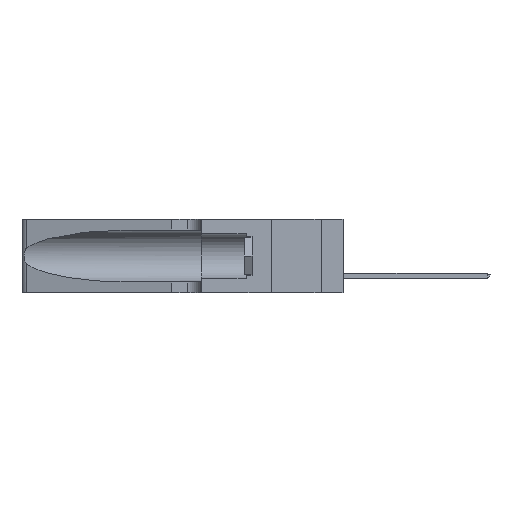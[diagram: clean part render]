
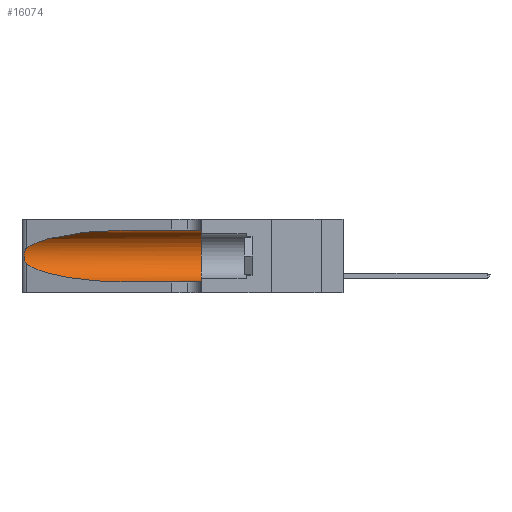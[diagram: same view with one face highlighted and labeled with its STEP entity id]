
A CAD part, left-side view. The second image highlights one B-rep face of the part: STEP entity #16074.
In plain terms, the highlighted cylindrical face has radius 3.308 mm (diameter 6.617 mm), a partial arc.
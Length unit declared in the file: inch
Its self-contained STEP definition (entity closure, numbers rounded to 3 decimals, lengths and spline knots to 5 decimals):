
#273 = CARTESIAN_POINT ( 'NONE',  ( 0.1305, 0.72297, 0.31525 ) ) ;
#564 = DIRECTION ( 'NONE',  ( 0., -1., 0. ) ) ;
#1654 = ORIENTED_EDGE ( 'NONE', *, *, #5495, .T. ) ;
#1999 = ORIENTED_EDGE ( 'NONE', *, *, #29885, .T. ) ;
#2245 = CARTESIAN_POINT ( 'NONE',  ( 0.25487, 1.22718, 0.14631 ) ) ;
#2535 = DIRECTION ( 'NONE',  ( 0., 0., 1. ) ) ;
#2566 = VERTEX_POINT ( 'NONE', #273 ) ;
#2699 = FACE_OUTER_BOUND ( 'NONE', #11051, .T. ) ;
#2924 = ORIENTED_EDGE ( 'NONE', *, *, #5559, .T. ) ;
#2955 = B_SPLINE_CURVE_WITH_KNOTS ( 'NONE', 3,
 ( #9701, #29972, #27235, #32277, #24946, #12218, #29869, #29764, #32486, #17508, #22674, #14862, #32379, #2245 ),
 .UNSPECIFIED., .F., .F.,
 ( 4, 2, 2, 2, 2, 2, 4 ),
 ( 0., 0.00027, 0.00053, 0.00107, 0.0016, 0.00187, 0.00214 ),
 .UNSPECIFIED. ) ;
#3397 = VERTEX_POINT ( 'NONE', #14533 ) ;
#4637 = EDGE_CURVE ( 'NONE', #3397, #16923, #11590, .T. ) ;
#5464 = CARTESIAN_POINT ( 'NONE',  ( 0.1305, 1.61858, 0.05475 ) ) ;
#5495 = EDGE_CURVE ( 'NONE', #12617, #23636, #2955, .T. ) ;
#5559 = EDGE_CURVE ( 'NONE', #23636, #8234, #9598, .T. ) ;
#6628 = EDGE_CURVE ( 'NONE', #2566, #12617, #17271, .T. ) ;
#6962 = CARTESIAN_POINT ( 'NONE',  ( 0.25487, 1.22718, 0.14631 ) ) ;
#7368 = ORIENTED_EDGE ( 'NONE', *, *, #6628, .T. ) ;
#8213 = VECTOR ( 'NONE', #564, 39.37008 ) ;
#8224 = LINE ( 'NONE', #31324, #26681 ) ;
#8234 = VERTEX_POINT ( 'NONE', #17272 ) ;
#8596 = ORIENTED_EDGE ( 'NONE', *, *, #4637, .F. ) ;
#8785 = CARTESIAN_POINT ( 'NONE',  ( 0.1305, 1.61858, 0.185 ) ) ;
#9102 = CARTESIAN_POINT ( 'NONE',  ( 0.25487, 1.22718, 0.22369 ) ) ;
#9598 =( BOUNDED_CURVE ( )  B_SPLINE_CURVE ( 3, ( #6962, #16991, #24649, #24552 ),
 .UNSPECIFIED., .F., .T. ) 
 B_SPLINE_CURVE_WITH_KNOTS ( ( 4, 4 ),
 ( 3.44316, 4.71239 ),
 .UNSPECIFIED. ) 
 CURVE ( )  GEOMETRIC_REPRESENTATION_ITEM ( )  RATIONAL_B_SPLINE_CURVE ( ( 1., 0.87, 0.87, 1. ) ) 
 REPRESENTATION_ITEM ( '' )  );
#9701 = CARTESIAN_POINT ( 'NONE',  ( 0.25487, 1.22718, 0.22369 ) ) ;
#11051 = EDGE_LOOP ( 'NONE', ( #7368, #1654, #2924, #1999, #8596, #26667 ) ) ;
#11590 = CIRCLE ( 'NONE', #21489, 0.13025 ) ;
#12218 = CARTESIAN_POINT ( 'NONE',  ( 0.26018, 1.23835, 0.19895 ) ) ;
#12264 = CARTESIAN_POINT ( 'NONE',  ( 0.2373, 1.15595, 0.28018 ) ) ;
#12617 = VERTEX_POINT ( 'NONE', #29669 ) ;
#14064 = DIRECTION ( 'NONE',  ( 0., 0., -1. ) ) ;
#14533 = CARTESIAN_POINT ( 'NONE',  ( 0.1305, 0.35, 0.31525 ) ) ;
#14862 = CARTESIAN_POINT ( 'NONE',  ( 0.25639, 1.23186, 0.15144 ) ) ;
#14901 = LINE ( 'NONE', #5464, #8213 ) ;
#15504 = EDGE_CURVE ( 'NONE', #2566, #3397, #8224, .T. ) ;
#16074 = ADVANCED_FACE ( 'NONE', ( #2699 ), #27773, .F. ) ;
#16923 = VERTEX_POINT ( 'NONE', #26718 ) ;
#16991 = CARTESIAN_POINT ( 'NONE',  ( 0.2373, 1.15595, 0.08982 ) ) ;
#17271 =( BOUNDED_CURVE ( )  B_SPLINE_CURVE ( 3, ( #24604, #31240, #12264, #9102 ),
 .UNSPECIFIED., .F., .T. ) 
 B_SPLINE_CURVE_WITH_KNOTS ( ( 4, 4 ),
 ( 1.5708, 2.84003 ),
 .UNSPECIFIED. ) 
 CURVE ( )  GEOMETRIC_REPRESENTATION_ITEM ( )  RATIONAL_B_SPLINE_CURVE ( ( 1., 0.87, 0.87, 1. ) ) 
 REPRESENTATION_ITEM ( '' )  );
#17272 = CARTESIAN_POINT ( 'NONE',  ( 0.1305, 0.72297, 0.05475 ) ) ;
#17508 = CARTESIAN_POINT ( 'NONE',  ( 0.25856, 1.23593, 0.16098 ) ) ;
#17803 = DIRECTION ( 'NONE',  ( 0., 1., 0. ) ) ;
#18982 = DIRECTION ( 'NONE',  ( 0., -1., 0. ) ) ;
#21489 = AXIS2_PLACEMENT_3D ( 'NONE', #30247, #17803, #2535 ) ;
#22674 = CARTESIAN_POINT ( 'NONE',  ( 0.25789, 1.23486, 0.15765 ) ) ;
#23636 = VERTEX_POINT ( 'NONE', #26754 ) ;
#24552 = CARTESIAN_POINT ( 'NONE',  ( 0.1305, 0.72297, 0.05475 ) ) ;
#24604 = CARTESIAN_POINT ( 'NONE',  ( 0.1305, 0.72297, 0.31525 ) ) ;
#24649 = CARTESIAN_POINT ( 'NONE',  ( 0.18966, 0.96281, 0.05475 ) ) ;
#24946 = CARTESIAN_POINT ( 'NONE',  ( 0.25854, 1.2359, 0.20912 ) ) ;
#25058 = AXIS2_PLACEMENT_3D ( 'NONE', #8785, #28850, #14064 ) ;
#26667 = ORIENTED_EDGE ( 'NONE', *, *, #15504, .F. ) ;
#26681 = VECTOR ( 'NONE', #18982, 39.37008 ) ;
#26718 = CARTESIAN_POINT ( 'NONE',  ( 0.1305, 0.35, 0.05475 ) ) ;
#26754 = CARTESIAN_POINT ( 'NONE',  ( 0.25487, 1.22718, 0.14631 ) ) ;
#27235 = CARTESIAN_POINT ( 'NONE',  ( 0.25639, 1.23184, 0.21858 ) ) ;
#27773 = CYLINDRICAL_SURFACE ( 'NONE', #25058, 0.13025 ) ;
#28850 = DIRECTION ( 'NONE',  ( 0., -1., 0. ) ) ;
#29669 = CARTESIAN_POINT ( 'NONE',  ( 0.25487, 1.22718, 0.22369 ) ) ;
#29764 = CARTESIAN_POINT ( 'NONE',  ( 0.26075, 1.23896, 0.178 ) ) ;
#29869 = CARTESIAN_POINT ( 'NONE',  ( 0.26075, 1.23896, 0.19203 ) ) ;
#29885 = EDGE_CURVE ( 'NONE', #8234, #16923, #14901, .T. ) ;
#29972 = CARTESIAN_POINT ( 'NONE',  ( 0.25555, 1.22994, 0.2215 ) ) ;
#30247 = CARTESIAN_POINT ( 'NONE',  ( 0.1305, 0.35, 0.185 ) ) ;
#31240 = CARTESIAN_POINT ( 'NONE',  ( 0.18966, 0.96281, 0.31525 ) ) ;
#31324 = CARTESIAN_POINT ( 'NONE',  ( 0.1305, 1.61858, 0.31525 ) ) ;
#32277 = CARTESIAN_POINT ( 'NONE',  ( 0.25787, 1.23484, 0.2124 ) ) ;
#32379 = CARTESIAN_POINT ( 'NONE',  ( 0.25555, 1.22993, 0.14849 ) ) ;
#32486 = CARTESIAN_POINT ( 'NONE',  ( 0.26017, 1.23833, 0.17102 ) ) ;
